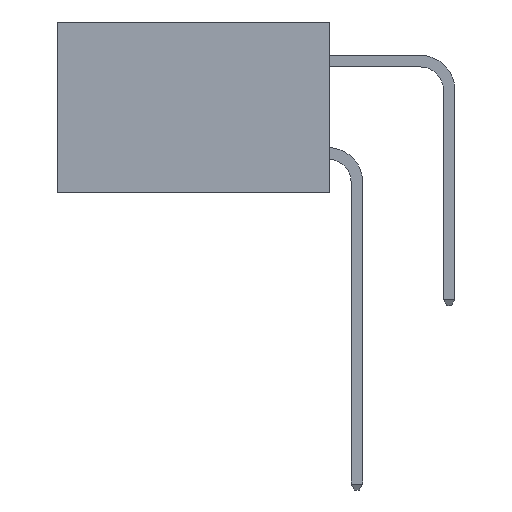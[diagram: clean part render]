
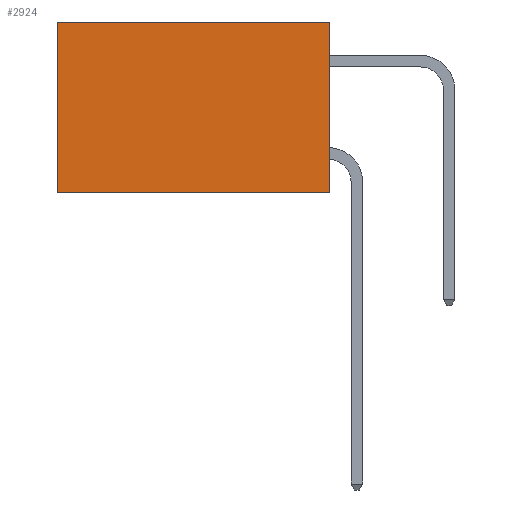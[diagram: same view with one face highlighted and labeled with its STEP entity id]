
A CAD part, left-side view. The second image highlights one B-rep face of the part: STEP entity #2924.
In plain terms, the highlighted planar face has unit normal (-1, 0, 0).
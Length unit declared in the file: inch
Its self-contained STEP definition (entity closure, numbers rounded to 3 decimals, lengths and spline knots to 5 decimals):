
#716 = LINE ( 'NONE', #3516, #5560 ) ;
#955 = DIRECTION ( 'NONE',  ( 0., 0., -1. ) ) ;
#1082 = CARTESIAN_POINT ( 'NONE',  ( 0.277, 0., 0. ) ) ;
#1461 = EDGE_CURVE ( 'NONE', #5236, #3736, #11638, .T. ) ;
#1536 = ORIENTED_EDGE ( 'NONE', *, *, #1461, .F. ) ;
#2566 = ORIENTED_EDGE ( 'NONE', *, *, #4755, .T. ) ;
#2849 = VERTEX_POINT ( 'NONE', #6496 ) ;
#2924 = ADVANCED_FACE ( 'NONE', ( #11085 ), #9685, .F. ) ;
#3191 = CARTESIAN_POINT ( 'NONE',  ( 0.277, 0., -0.37 ) ) ;
#3233 = DIRECTION ( 'NONE',  ( 0., 1., 0. ) ) ;
#3516 = CARTESIAN_POINT ( 'NONE',  ( 0.277, 0., 0. ) ) ;
#3736 = VERTEX_POINT ( 'NONE', #8919 ) ;
#3894 = VERTEX_POINT ( 'NONE', #1082 ) ;
#4217 = EDGE_CURVE ( 'NONE', #3894, #2849, #716, .T. ) ;
#4294 = DIRECTION ( 'NONE',  ( 0., 0., -1. ) ) ;
#4755 = EDGE_CURVE ( 'NONE', #2849, #3736, #11399, .T. ) ;
#4756 = DIRECTION ( 'NONE',  ( 0., 0., -1. ) ) ;
#5236 = VERTEX_POINT ( 'NONE', #11448 ) ;
#5560 = VECTOR ( 'NONE', #9143, 39.37008 ) ;
#6024 = EDGE_LOOP ( 'NONE', ( #2566, #1536, #9412, #7235 ) ) ;
#6496 = CARTESIAN_POINT ( 'NONE',  ( 0.277, 0.59, 0. ) ) ;
#6615 = DIRECTION ( 'NONE',  ( 1., 0., 0. ) ) ;
#6864 = EDGE_CURVE ( 'NONE', #3894, #5236, #10866, .T. ) ;
#7235 = ORIENTED_EDGE ( 'NONE', *, *, #4217, .T. ) ;
#7260 = AXIS2_PLACEMENT_3D ( 'NONE', #9995, #6615, #4756 ) ;
#8229 = VECTOR ( 'NONE', #955, 39.37008 ) ;
#8919 = CARTESIAN_POINT ( 'NONE',  ( 0.277, 0.59, -0.37 ) ) ;
#9143 = DIRECTION ( 'NONE',  ( 0., 1., 0. ) ) ;
#9412 = ORIENTED_EDGE ( 'NONE', *, *, #6864, .F. ) ;
#9428 = VECTOR ( 'NONE', #3233, 39.37008 ) ;
#9685 = PLANE ( 'NONE',  #7260 ) ;
#9995 = CARTESIAN_POINT ( 'NONE',  ( 0.277, 0., -0.37 ) ) ;
#10723 = CARTESIAN_POINT ( 'NONE',  ( 0.277, 0.59, -0.37 ) ) ;
#10866 = LINE ( 'NONE', #11972, #8229 ) ;
#11085 = FACE_OUTER_BOUND ( 'NONE', #6024, .T. ) ;
#11137 = VECTOR ( 'NONE', #4294, 39.37008 ) ;
#11399 = LINE ( 'NONE', #10723, #11137 ) ;
#11448 = CARTESIAN_POINT ( 'NONE',  ( 0.277, 0., -0.37 ) ) ;
#11638 = LINE ( 'NONE', #3191, #9428 ) ;
#11972 = CARTESIAN_POINT ( 'NONE',  ( 0.277, 0., -0.37 ) ) ;
